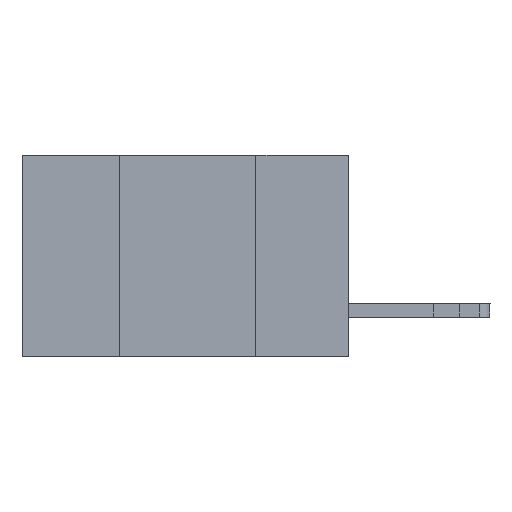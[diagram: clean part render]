
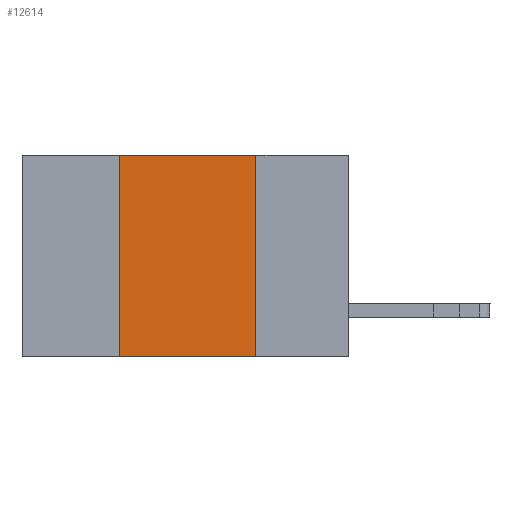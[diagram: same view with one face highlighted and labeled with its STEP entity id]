
A CAD part, left-side view. The second image highlights one B-rep face of the part: STEP entity #12614.
In plain terms, the highlighted planar face has unit normal (-1, 0, 0).
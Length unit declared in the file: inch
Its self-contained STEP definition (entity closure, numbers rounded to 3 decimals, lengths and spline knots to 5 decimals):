
#280 = VECTOR ( 'NONE', #6912, 39.37008 ) ;
#325 = LINE ( 'NONE', #9512, #13220 ) ;
#393 = CARTESIAN_POINT ( 'NONE',  ( 0., 0.6, 0. ) ) ;
#1011 = LINE ( 'NONE', #13965, #280 ) ;
#1413 = FACE_OUTER_BOUND ( 'NONE', #5306, .T. ) ;
#1454 = EDGE_CURVE ( 'NONE', #4197, #13505, #12304, .T. ) ;
#2255 = EDGE_CURVE ( 'NONE', #13987, #13505, #325, .T. ) ;
#3982 = DIRECTION ( 'NONE',  ( 0., -1., 0. ) ) ;
#4197 = VERTEX_POINT ( 'NONE', #12509 ) ;
#4228 = LINE ( 'NONE', #393, #13761 ) ;
#4447 = ORIENTED_EDGE ( 'NONE', *, *, #2255, .T. ) ;
#4731 = VERTEX_POINT ( 'NONE', #6991 ) ;
#4828 = DIRECTION ( 'NONE',  ( 0., -1., 0. ) ) ;
#5011 = VECTOR ( 'NONE', #5176, 39.37008 ) ;
#5176 = DIRECTION ( 'NONE',  ( 0., 0., -1. ) ) ;
#5306 = EDGE_LOOP ( 'NONE', ( #9388, #11678, #9267, #4447 ) ) ;
#5626 = CARTESIAN_POINT ( 'NONE',  ( 0., 0.17, -0.37 ) ) ;
#6279 = CARTESIAN_POINT ( 'NONE',  ( 0., 0.17, 0. ) ) ;
#6751 = CARTESIAN_POINT ( 'NONE',  ( 0., 0.6, 0. ) ) ;
#6912 = DIRECTION ( 'NONE',  ( 0., 0., 1. ) ) ;
#6991 = CARTESIAN_POINT ( 'NONE',  ( 0., 0.42, 0. ) ) ;
#7901 = PLANE ( 'NONE',  #11787 ) ;
#8451 = CARTESIAN_POINT ( 'NONE',  ( 0., 0.42, -0.37 ) ) ;
#9267 = ORIENTED_EDGE ( 'NONE', *, *, #10373, .F. ) ;
#9388 = ORIENTED_EDGE ( 'NONE', *, *, #1454, .F. ) ;
#9512 = CARTESIAN_POINT ( 'NONE',  ( 0., 0.6, -0.37 ) ) ;
#10373 = EDGE_CURVE ( 'NONE', #13987, #4731, #1011, .T. ) ;
#11388 = DIRECTION ( 'NONE',  ( 1., 0., 0. ) ) ;
#11470 = EDGE_CURVE ( 'NONE', #4731, #4197, #4228, .T. ) ;
#11678 = ORIENTED_EDGE ( 'NONE', *, *, #11470, .F. ) ;
#11787 = AXIS2_PLACEMENT_3D ( 'NONE', #6751, #11388, #13585 ) ;
#12304 = LINE ( 'NONE', #6279, #5011 ) ;
#12509 = CARTESIAN_POINT ( 'NONE',  ( 0., 0.17, 0. ) ) ;
#12614 = ADVANCED_FACE ( 'NONE', ( #1413 ), #7901, .F. ) ;
#13220 = VECTOR ( 'NONE', #4828, 39.37008 ) ;
#13505 = VERTEX_POINT ( 'NONE', #5626 ) ;
#13585 = DIRECTION ( 'NONE',  ( 0., 0., -1. ) ) ;
#13761 = VECTOR ( 'NONE', #3982, 39.37008 ) ;
#13965 = CARTESIAN_POINT ( 'NONE',  ( 0., 0.42, 0. ) ) ;
#13987 = VERTEX_POINT ( 'NONE', #8451 ) ;
